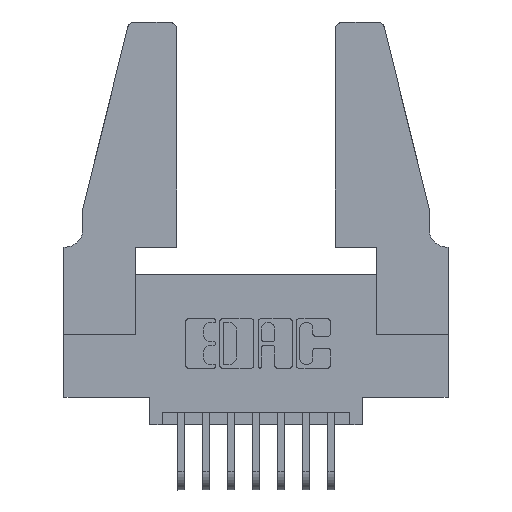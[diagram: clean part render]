
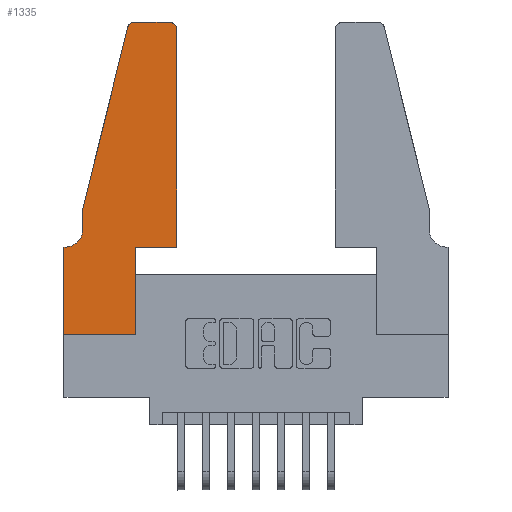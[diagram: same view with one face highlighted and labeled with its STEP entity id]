
A CAD part, top view. The second image highlights one B-rep face of the part: STEP entity #1335.
In plain terms, the highlighted planar face has unit normal (0, 0, 1).
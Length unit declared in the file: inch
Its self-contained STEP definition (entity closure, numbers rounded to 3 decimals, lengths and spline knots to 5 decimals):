
#31 = CARTESIAN_POINT ( 'NONE',  ( 0.284, 1.25, 0.37 ) ) ;
#154 = VECTOR ( 'NONE', #11296, 39.37008 ) ;
#223 = EDGE_CURVE ( 'NONE', #640, #5179, #8273, .T. ) ;
#305 = AXIS2_PLACEMENT_3D ( 'NONE', #953, #1178, #1509 ) ;
#351 = LINE ( 'NONE', #11325, #154 ) ;
#392 = EDGE_CURVE ( 'NONE', #6890, #1033, #6078, .T. ) ;
#397 = VECTOR ( 'NONE', #10461, 39.37008 ) ;
#503 = LINE ( 'NONE', #8912, #397 ) ;
#551 = DIRECTION ( 'NONE',  ( 0., 0., 1. ) ) ;
#588 = CARTESIAN_POINT ( 'NONE',  ( 0.284, 1.22, 0.37 ) ) ;
#640 = VERTEX_POINT ( 'NONE', #31 ) ;
#804 = DIRECTION ( 'NONE',  ( 1., 0., 0. ) ) ;
#914 = VERTEX_POINT ( 'NONE', #10218 ) ;
#953 = CARTESIAN_POINT ( 'NONE',  ( 0.0055, 0.42, 0.37 ) ) ;
#1033 = VERTEX_POINT ( 'NONE', #5604 ) ;
#1178 = DIRECTION ( 'NONE',  ( 0., 0., -1. ) ) ;
#1335 = ADVANCED_FACE ( 'NONE', ( #11773 ), #4537, .T. ) ;
#1509 = DIRECTION ( 'NONE',  ( -1., 0., 0. ) ) ;
#1866 = CIRCLE ( 'NONE', #5162, 0.03 ) ;
#2033 = AXIS2_PLACEMENT_3D ( 'NONE', #588, #551, #2869 ) ;
#2079 = VERTEX_POINT ( 'NONE', #2396 ) ;
#2363 = VERTEX_POINT ( 'NONE', #5695 ) ;
#2396 = CARTESIAN_POINT ( 'NONE',  ( 0.4505, 0.35, 0.37 ) ) ;
#2869 = DIRECTION ( 'NONE',  ( 1., 0., 0. ) ) ;
#3084 = ORIENTED_EDGE ( 'NONE', *, *, #5844, .T. ) ;
#3129 = DIRECTION ( 'NONE',  ( -0.239, -0.971, 0. ) ) ;
#3484 = ORIENTED_EDGE ( 'NONE', *, *, #223, .T. ) ;
#3504 = CARTESIAN_POINT ( 'NONE',  ( 0.2865, 0., 0.37 ) ) ;
#3629 = CARTESIAN_POINT ( 'NONE',  ( 0.0755, 0.42, 0.37 ) ) ;
#3682 = ORIENTED_EDGE ( 'NONE', *, *, #11255, .T. ) ;
#3869 = DIRECTION ( 'NONE',  ( 0., 1., 0. ) ) ;
#4109 = CARTESIAN_POINT ( 'NONE',  ( 0.4505, 1.22, 0.37 ) ) ;
#4319 = CARTESIAN_POINT ( 'NONE',  ( 0., 0., 0.37 ) ) ;
#4537 = PLANE ( 'NONE',  #9419 ) ;
#4787 = LINE ( 'NONE', #9208, #4948 ) ;
#4795 = ORIENTED_EDGE ( 'NONE', *, *, #4912, .T. ) ;
#4799 = CARTESIAN_POINT ( 'NONE',  ( 0.0755, 0.5, 0.37 ) ) ;
#4912 = EDGE_CURVE ( 'NONE', #914, #6890, #10427, .T. ) ;
#4946 = ORIENTED_EDGE ( 'NONE', *, *, #392, .T. ) ;
#4948 = VECTOR ( 'NONE', #3129, 39.37008 ) ;
#5162 = AXIS2_PLACEMENT_3D ( 'NONE', #12210, #7677, #804 ) ;
#5173 = ORIENTED_EDGE ( 'NONE', *, *, #7649, .T. ) ;
#5179 = VERTEX_POINT ( 'NONE', #11554 ) ;
#5180 = VERTEX_POINT ( 'NONE', #6695 ) ;
#5559 = EDGE_CURVE ( 'NONE', #7229, #10740, #7491, .T. ) ;
#5604 = CARTESIAN_POINT ( 'NONE',  ( 0.0055, 0.35, 0.37 ) ) ;
#5682 = ORIENTED_EDGE ( 'NONE', *, *, #5894, .T. ) ;
#5695 = CARTESIAN_POINT ( 'NONE',  ( 0., 0.35, 0.37 ) ) ;
#5844 = EDGE_CURVE ( 'NONE', #6626, #640, #503, .T. ) ;
#5894 = EDGE_CURVE ( 'NONE', #2363, #7229, #351, .T. ) ;
#5911 = ORIENTED_EDGE ( 'NONE', *, *, #5559, .T. ) ;
#5950 = DIRECTION ( 'NONE',  ( 0., -1., 0. ) ) ;
#6078 = CIRCLE ( 'NONE', #305, 0.07 ) ;
#6338 = ORIENTED_EDGE ( 'NONE', *, *, #8880, .T. ) ;
#6407 = DIRECTION ( 'NONE',  ( 1., 0., 0. ) ) ;
#6504 = VECTOR ( 'NONE', #6715, 39.37008 ) ;
#6626 = VERTEX_POINT ( 'NONE', #6648 ) ;
#6648 = CARTESIAN_POINT ( 'NONE',  ( 0.4205, 1.25, 0.37 ) ) ;
#6695 = CARTESIAN_POINT ( 'NONE',  ( 0.2865, 0.35, 0.37 ) ) ;
#6703 = LINE ( 'NONE', #12241, #6504 ) ;
#6715 = DIRECTION ( 'NONE',  ( -1., 0., 0. ) ) ;
#6890 = VERTEX_POINT ( 'NONE', #3629 ) ;
#7229 = VERTEX_POINT ( 'NONE', #7294 ) ;
#7294 = CARTESIAN_POINT ( 'NONE',  ( 0., 0., 0.37 ) ) ;
#7420 = VECTOR ( 'NONE', #9936, 39.37008 ) ;
#7491 = LINE ( 'NONE', #4319, #7420 ) ;
#7649 = EDGE_CURVE ( 'NONE', #1033, #2363, #6703, .T. ) ;
#7677 = DIRECTION ( 'NONE',  ( 0., 0., 1. ) ) ;
#8273 = CIRCLE ( 'NONE', #2033, 0.03 ) ;
#8406 = EDGE_CURVE ( 'NONE', #2079, #9007, #11543, .T. ) ;
#8563 = CARTESIAN_POINT ( 'NONE',  ( 0., 0.35, 0.37 ) ) ;
#8566 = ORIENTED_EDGE ( 'NONE', *, *, #9086, .T. ) ;
#8880 = EDGE_CURVE ( 'NONE', #10740, #5180, #10481, .T. ) ;
#8912 = CARTESIAN_POINT ( 'NONE',  ( 0.2605, 1.25, 0.37 ) ) ;
#9007 = VERTEX_POINT ( 'NONE', #4109 ) ;
#9072 = CARTESIAN_POINT ( 'NONE',  ( 0.4505, 0.35, 0.37 ) ) ;
#9086 = EDGE_CURVE ( 'NONE', #5180, #2079, #9896, .T. ) ;
#9208 = CARTESIAN_POINT ( 'NONE',  ( 0.0755, 0.5, 0.37 ) ) ;
#9419 = AXIS2_PLACEMENT_3D ( 'NONE', #8563, #10985, #10576 ) ;
#9801 = VECTOR ( 'NONE', #6407, 39.37008 ) ;
#9896 = LINE ( 'NONE', #9072, #9801 ) ;
#9927 = ORIENTED_EDGE ( 'NONE', *, *, #8406, .T. ) ;
#9936 = DIRECTION ( 'NONE',  ( 1., 0., 0. ) ) ;
#9953 = DIRECTION ( 'NONE',  ( 0., 1., 0. ) ) ;
#9981 = ORIENTED_EDGE ( 'NONE', *, *, #11968, .T. ) ;
#9984 = CARTESIAN_POINT ( 'NONE',  ( 0.4505, 0.35, 0.37 ) ) ;
#10218 = CARTESIAN_POINT ( 'NONE',  ( 0.0755, 0.5, 0.37 ) ) ;
#10259 = EDGE_LOOP ( 'NONE', ( #3084, #3484, #3682, #4795, #4946, #5173, #5682, #5911, #6338, #8566, #9927, #9981 ) ) ;
#10325 = VECTOR ( 'NONE', #5950, 39.37008 ) ;
#10427 = LINE ( 'NONE', #4799, #10325 ) ;
#10461 = DIRECTION ( 'NONE',  ( -1., 0., 0. ) ) ;
#10481 = LINE ( 'NONE', #11887, #10544 ) ;
#10544 = VECTOR ( 'NONE', #3869, 39.37008 ) ;
#10576 = DIRECTION ( 'NONE',  ( 1., 0., 0. ) ) ;
#10740 = VERTEX_POINT ( 'NONE', #3504 ) ;
#10985 = DIRECTION ( 'NONE',  ( 0., 0., 1. ) ) ;
#11255 = EDGE_CURVE ( 'NONE', #5179, #914, #4787, .T. ) ;
#11296 = DIRECTION ( 'NONE',  ( 0., -1., 0. ) ) ;
#11325 = CARTESIAN_POINT ( 'NONE',  ( 0., 0., 0.37 ) ) ;
#11535 = VECTOR ( 'NONE', #9953, 39.37008 ) ;
#11543 = LINE ( 'NONE', #9984, #11535 ) ;
#11554 = CARTESIAN_POINT ( 'NONE',  ( 0.25487, 1.22718, 0.37 ) ) ;
#11773 = FACE_OUTER_BOUND ( 'NONE', #10259, .T. ) ;
#11887 = CARTESIAN_POINT ( 'NONE',  ( 0.2865, 0.35, 0.37 ) ) ;
#11968 = EDGE_CURVE ( 'NONE', #9007, #6626, #1866, .T. ) ;
#12210 = CARTESIAN_POINT ( 'NONE',  ( 0.4205, 1.22, 0.37 ) ) ;
#12241 = CARTESIAN_POINT ( 'NONE',  ( 0.0755, 0.35, 0.37 ) ) ;
